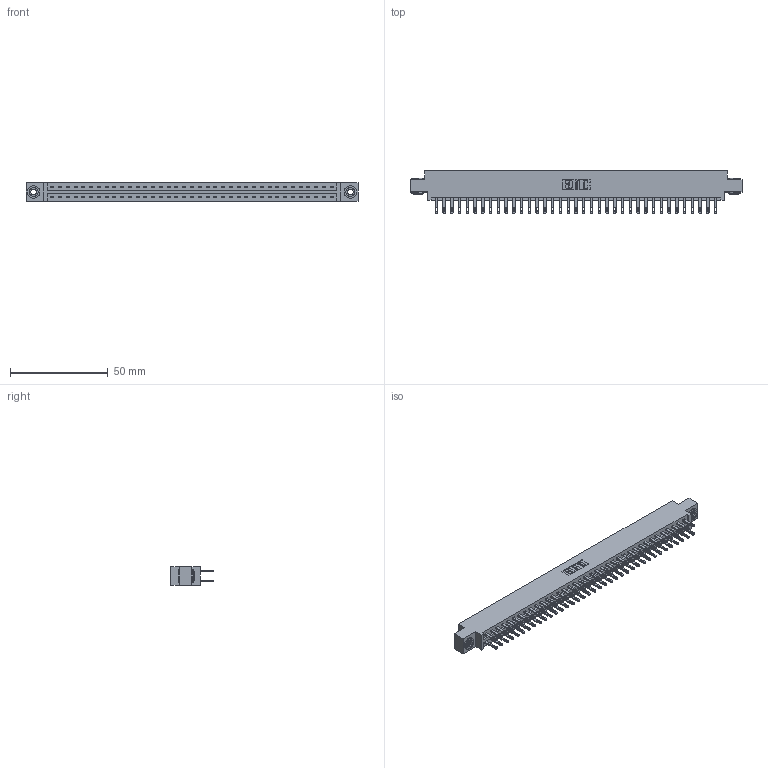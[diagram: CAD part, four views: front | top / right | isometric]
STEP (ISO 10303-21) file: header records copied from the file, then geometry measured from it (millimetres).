
FILE_DESCRIPTION (( 'STEP AP203' ), '1' );
FILE_NAME ('337-074-500-803.STEP', '2018-08-11T16:19:59', ( '' ), ( '' ), 'SwSTEP 2.0', 'SolidWorks 2016', '' );
FILE_SCHEMA (( 'CONFIG_CONTROL_DESIGN' ));
Length unit declared in the file: inch
Products named in the file (4): 345-250-002_345-250-002-102; 337-074-500-803; 337 Part_0.170 Offset - 0.156 Dia-TH; 345-292-001_345-293-100
Assembly tree (77 placements, depth 2):
  337-074-500-803
    337 Part_0.170 Offset - 0.156 Dia-TH
    345-292-001_345-293-100  x74
    345-250-002_345-250-002-102  x2
Bounding box: 169.62 x 21.85 x 9.4 mm (x, y, z)
Volume: 17937.5 mm3; surface area: 21383.1 mm2
Topology: 77 solids, 77 shells, 3856 faces, 11721 edges, 7810 vertices
Faces by surface type: plane 2452, cylinder 1396, cone 8
Entity records: 30046 total; most frequent: CARTESIAN_POINT 5041, ORIENTED_EDGE 4970, DIRECTION 4331, EDGE_CURVE 2485, VECTOR 2329, LINE 2329, VERTEX_POINT 1654, AXIS2_PLACEMENT_3D 1001
